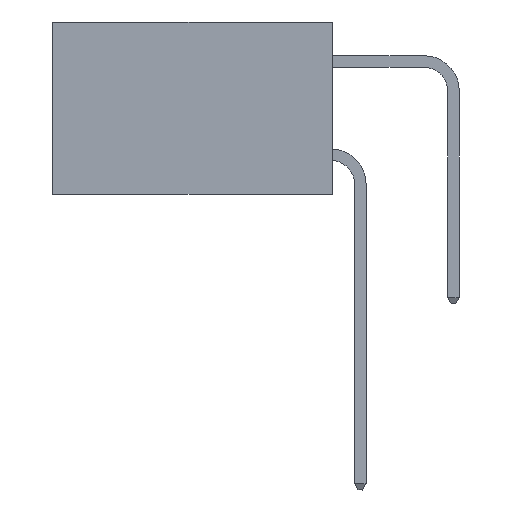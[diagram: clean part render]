
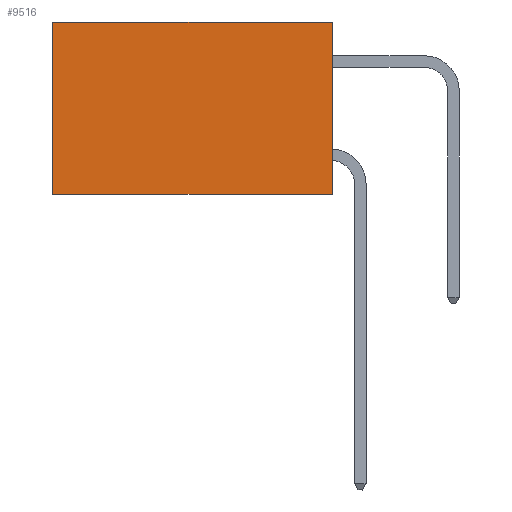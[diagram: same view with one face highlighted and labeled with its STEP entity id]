
A CAD part, left-side view. The second image highlights one B-rep face of the part: STEP entity #9516.
In plain terms, the highlighted planar face has unit normal (-1, 0, 0).
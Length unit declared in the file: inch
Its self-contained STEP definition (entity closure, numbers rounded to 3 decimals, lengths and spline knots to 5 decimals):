
#85 = EDGE_CURVE ( 'NONE', #12907, #19579, #15568, .T. ) ;
#193 = ORIENTED_EDGE ( 'NONE', *, *, #13542, .T. ) ;
#860 = CARTESIAN_POINT ( 'NONE',  ( 0.2615, 0.6, -0.37 ) ) ;
#1585 = PLANE ( 'NONE',  #2311 ) ;
#2311 = AXIS2_PLACEMENT_3D ( 'NONE', #11046, #18687, #3322 ) ;
#2348 = CARTESIAN_POINT ( 'NONE',  ( 0.2615, 0., -0.37 ) ) ;
#3322 = DIRECTION ( 'NONE',  ( 0., 0., -1. ) ) ;
#3747 = LINE ( 'NONE', #7049, #13887 ) ;
#3841 = VECTOR ( 'NONE', #13076, 39.37008 ) ;
#4098 = EDGE_LOOP ( 'NONE', ( #193, #17249, #10131, #7858 ) ) ;
#4913 = VECTOR ( 'NONE', #13970, 39.37008 ) ;
#5562 = EDGE_CURVE ( 'NONE', #11268, #6623, #19580, .T. ) ;
#6134 = CARTESIAN_POINT ( 'NONE',  ( 0.2615, 0., -0.37 ) ) ;
#6623 = VERTEX_POINT ( 'NONE', #860 ) ;
#7049 = CARTESIAN_POINT ( 'NONE',  ( 0.2615, 0.6, -0.37 ) ) ;
#7858 = ORIENTED_EDGE ( 'NONE', *, *, #85, .T. ) ;
#7868 = LINE ( 'NONE', #6134, #4913 ) ;
#9397 = FACE_OUTER_BOUND ( 'NONE', #4098, .T. ) ;
#9516 = ADVANCED_FACE ( 'NONE', ( #9397 ), #1585, .F. ) ;
#10131 = ORIENTED_EDGE ( 'NONE', *, *, #18693, .F. ) ;
#10703 = DIRECTION ( 'NONE',  ( 0., 1., 0. ) ) ;
#11046 = CARTESIAN_POINT ( 'NONE',  ( 0.2615, 0., -0.37 ) ) ;
#11126 = VECTOR ( 'NONE', #10703, 39.37008 ) ;
#11268 = VERTEX_POINT ( 'NONE', #2348 ) ;
#12907 = VERTEX_POINT ( 'NONE', #17289 ) ;
#13076 = DIRECTION ( 'NONE',  ( 0., 1., 0. ) ) ;
#13542 = EDGE_CURVE ( 'NONE', #19579, #6623, #3747, .T. ) ;
#13887 = VECTOR ( 'NONE', #16246, 39.37008 ) ;
#13970 = DIRECTION ( 'NONE',  ( 0., 0., -1. ) ) ;
#14011 = CARTESIAN_POINT ( 'NONE',  ( 0.2615, 0., 0. ) ) ;
#15372 = CARTESIAN_POINT ( 'NONE',  ( 0.2615, 0.6, 0. ) ) ;
#15568 = LINE ( 'NONE', #14011, #11126 ) ;
#16246 = DIRECTION ( 'NONE',  ( 0., 0., -1. ) ) ;
#16504 = CARTESIAN_POINT ( 'NONE',  ( 0.2615, 0., -0.37 ) ) ;
#17249 = ORIENTED_EDGE ( 'NONE', *, *, #5562, .F. ) ;
#17289 = CARTESIAN_POINT ( 'NONE',  ( 0.2615, 0., 0. ) ) ;
#18687 = DIRECTION ( 'NONE',  ( 1., 0., 0. ) ) ;
#18693 = EDGE_CURVE ( 'NONE', #12907, #11268, #7868, .T. ) ;
#19579 = VERTEX_POINT ( 'NONE', #15372 ) ;
#19580 = LINE ( 'NONE', #16504, #3841 ) ;
